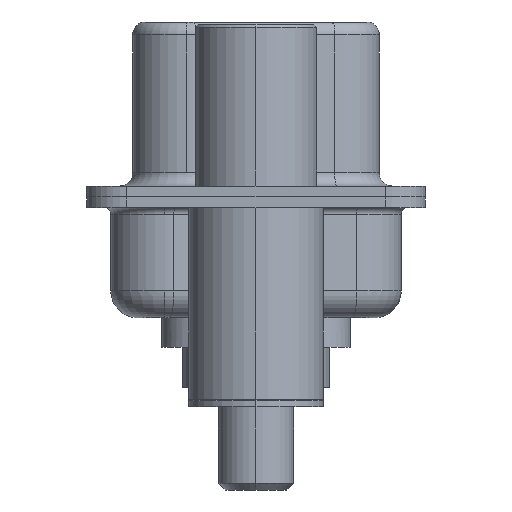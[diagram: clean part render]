
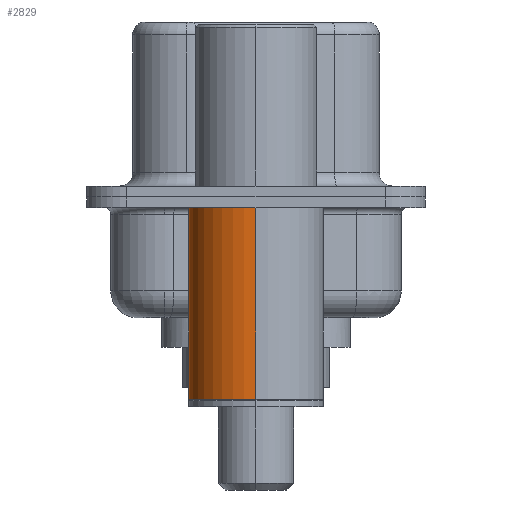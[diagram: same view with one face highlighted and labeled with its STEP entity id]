
A CAD part, left-side view. The second image highlights one B-rep face of the part: STEP entity #2829.
In plain terms, the highlighted cylindrical face has radius 2.5 mm (diameter 5 mm), a partial arc.
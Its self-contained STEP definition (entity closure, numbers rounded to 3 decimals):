
#738 = CARTESIAN_POINT ( 'NONE',  ( 2.5, 0., -0.4 ) ) ;
#1120 = DIRECTION ( 'NONE',  ( 0., 0., 1. ) ) ;
#2117 = ORIENTED_EDGE ( 'NONE', *, *, #15928, .F. ) ;
#2253 = EDGE_CURVE ( 'NONE', #15645, #13400, #14962, .T. ) ;
#2501 = DIRECTION ( 'NONE',  ( 0., 0., 1. ) ) ;
#2539 = ORIENTED_EDGE ( 'NONE', *, *, #12586, .T. ) ;
#2685 = CARTESIAN_POINT ( 'NONE',  ( -2.5, 0., 0.581 ) ) ;
#2829 = ADVANCED_FACE ( 'NONE', ( #13364 ), #6783, .T. ) ;
#3551 = CIRCLE ( 'NONE', #4760, 2.5 ) ;
#3608 = LINE ( 'NONE', #8075, #16056 ) ;
#3880 = VERTEX_POINT ( 'NONE', #15649 ) ;
#4760 = AXIS2_PLACEMENT_3D ( 'NONE', #9985, #2501, #11248 ) ;
#4829 = AXIS2_PLACEMENT_3D ( 'NONE', #8626, #1120, #9927 ) ;
#6373 = ORIENTED_EDGE ( 'NONE', *, *, #2253, .T. ) ;
#6783 = CYLINDRICAL_SURFACE ( 'NONE', #11078, 2.5 ) ;
#6904 = DIRECTION ( 'NONE',  ( 0., 0., 1. ) ) ;
#7098 = CARTESIAN_POINT ( 'NONE',  ( -2.5, 0., -7.525 ) ) ;
#8075 = CARTESIAN_POINT ( 'NONE',  ( 2.5, 0., 0.581 ) ) ;
#8325 = VECTOR ( 'NONE', #10810, 1000. ) ;
#8626 = CARTESIAN_POINT ( 'NONE',  ( 0., 0., -7.525 ) ) ;
#9927 = DIRECTION ( 'NONE',  ( 1., 0., 0. ) ) ;
#9985 = CARTESIAN_POINT ( 'NONE',  ( 0., 0., -0.4 ) ) ;
#10810 = DIRECTION ( 'NONE',  ( 0., 0., 1. ) ) ;
#10975 = ORIENTED_EDGE ( 'NONE', *, *, #11769, .F. ) ;
#11078 = AXIS2_PLACEMENT_3D ( 'NONE', #13734, #13784, #13767 ) ;
#11192 = CIRCLE ( 'NONE', #4829, 2.5 ) ;
#11248 = DIRECTION ( 'NONE',  ( 1., 0., 0. ) ) ;
#11769 = EDGE_CURVE ( 'NONE', #3880, #15623, #3608, .T. ) ;
#12586 = EDGE_CURVE ( 'NONE', #3880, #15645, #11192, .T. ) ;
#12653 = CARTESIAN_POINT ( 'NONE',  ( -2.5, 0., -0.4 ) ) ;
#13141 = EDGE_LOOP ( 'NONE', ( #2539, #6373, #2117, #10975 ) ) ;
#13364 = FACE_OUTER_BOUND ( 'NONE', #13141, .T. ) ;
#13400 = VERTEX_POINT ( 'NONE', #12653 ) ;
#13734 = CARTESIAN_POINT ( 'NONE',  ( 0., 0., 0.581 ) ) ;
#13767 = DIRECTION ( 'NONE',  ( 1., 0., 0. ) ) ;
#13784 = DIRECTION ( 'NONE',  ( 0., 0., 1. ) ) ;
#14962 = LINE ( 'NONE', #2685, #8325 ) ;
#15623 = VERTEX_POINT ( 'NONE', #738 ) ;
#15645 = VERTEX_POINT ( 'NONE', #7098 ) ;
#15649 = CARTESIAN_POINT ( 'NONE',  ( 2.5, 0., -7.525 ) ) ;
#15928 = EDGE_CURVE ( 'NONE', #15623, #13400, #3551, .T. ) ;
#16056 = VECTOR ( 'NONE', #6904, 1000. ) ;
